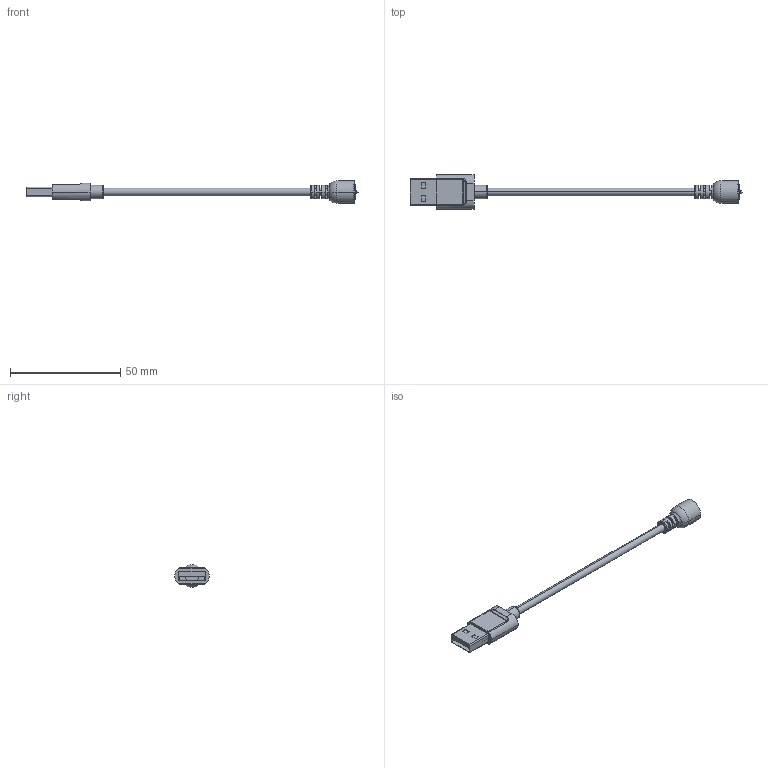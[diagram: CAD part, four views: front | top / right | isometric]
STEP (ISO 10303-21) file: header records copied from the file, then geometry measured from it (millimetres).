
FILE_DESCRIPTION (( 'STEP AP203' ), '1' );
FILE_NAME ('MCM-Q00-0E2-2P14-BH0.STEP', '2025-09-10T12:45:38', ( '' ), ( '' ), 'SwSTEP 2.0', 'SolidWorks 2023', '' );
FILE_SCHEMA (( 'CONFIG_CONTROL_DESIGN' ));
Length unit declared in the file: millimetre
Products named in the file (1): MCM-Q00-0E2-2P14-BH0
Bounding box: 150.4 x 15.8 x 10.4 mm (x, y, z)
Surface area: 3784.5 mm2 (no closed solid volume)
Topology: 0 solids, 12 shells, 169 faces, 467 edges, 315 vertices
Faces by surface type: plane 85, cylinder 52, torus 16, bspline 12, cone 2, sphere 2
Entity records: 5557 total; most frequent: CARTESIAN_POINT 1154, DIRECTION 929, ORIENTED_EDGE 846, EDGE_CURVE 465, AXIS2_PLACEMENT_3D 330, VERTEX_POINT 315, LINE 269, VECTOR 269
